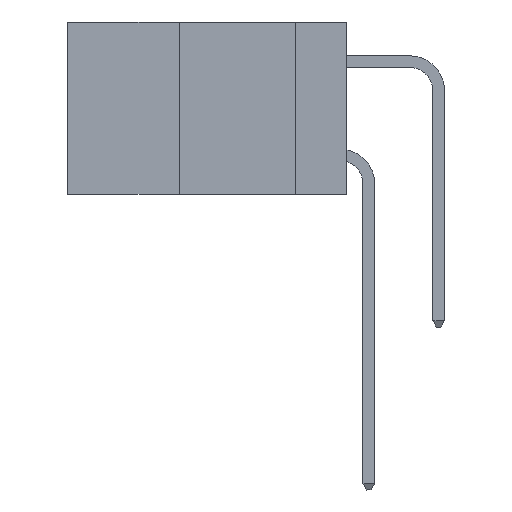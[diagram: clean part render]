
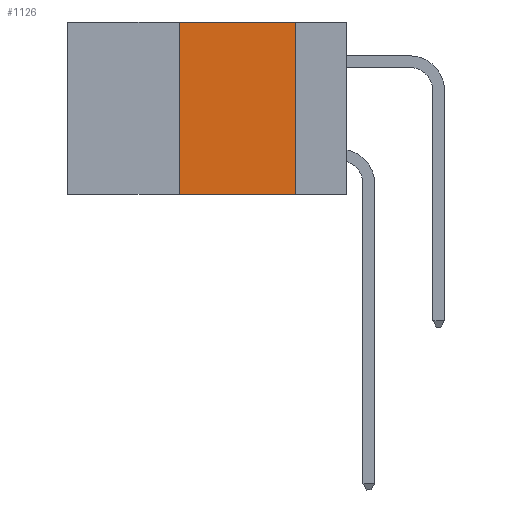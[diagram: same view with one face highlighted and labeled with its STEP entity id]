
A CAD part, left-side view. The second image highlights one B-rep face of the part: STEP entity #1126.
In plain terms, the highlighted planar face has unit normal (-1, 0, 0).
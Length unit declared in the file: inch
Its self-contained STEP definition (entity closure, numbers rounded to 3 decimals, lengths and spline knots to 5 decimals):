
#387 = CARTESIAN_POINT ( 'NONE',  ( 0., 0.6, 0. ) ) ;
#1126 = ADVANCED_FACE ( 'NONE', ( #11434 ), #13312, .F. ) ;
#2024 = VERTEX_POINT ( 'NONE', #13563 ) ;
#3400 = CARTESIAN_POINT ( 'NONE',  ( 0., 0.36, -0.37 ) ) ;
#3711 = DIRECTION ( 'NONE',  ( 0., 0., -1. ) ) ;
#4154 = EDGE_CURVE ( 'NONE', #9058, #19935, #14479, .T. ) ;
#4183 = VECTOR ( 'NONE', #19944, 39.37008 ) ;
#4853 = CARTESIAN_POINT ( 'NONE',  ( 0., 0.6, 0. ) ) ;
#5461 = DIRECTION ( 'NONE',  ( 1., 0., 0. ) ) ;
#5566 = EDGE_LOOP ( 'NONE', ( #8523, #20035, #20902, #6973 ) ) ;
#5877 = VECTOR ( 'NONE', #8380, 39.37008 ) ;
#6034 = VECTOR ( 'NONE', #18378, 39.37008 ) ;
#6973 = ORIENTED_EDGE ( 'NONE', *, *, #12761, .T. ) ;
#8380 = DIRECTION ( 'NONE',  ( 0., 0., 1. ) ) ;
#8500 = CARTESIAN_POINT ( 'NONE',  ( 0., 0.36, 0. ) ) ;
#8523 = ORIENTED_EDGE ( 'NONE', *, *, #13667, .F. ) ;
#8695 = LINE ( 'NONE', #387, #4183 ) ;
#9058 = VERTEX_POINT ( 'NONE', #3400 ) ;
#11434 = FACE_OUTER_BOUND ( 'NONE', #5566, .T. ) ;
#12340 = EDGE_CURVE ( 'NONE', #19935, #2024, #8695, .T. ) ;
#12685 = CARTESIAN_POINT ( 'NONE',  ( 0., 0.11, -0.37 ) ) ;
#12761 = EDGE_CURVE ( 'NONE', #9058, #17149, #17138, .T. ) ;
#13045 = DIRECTION ( 'NONE',  ( 0., -1., 0. ) ) ;
#13312 = PLANE ( 'NONE',  #15324 ) ;
#13563 = CARTESIAN_POINT ( 'NONE',  ( 0., 0.11, 0. ) ) ;
#13667 = EDGE_CURVE ( 'NONE', #2024, #17149, #18321, .T. ) ;
#14479 = LINE ( 'NONE', #8500, #5877 ) ;
#15232 = CARTESIAN_POINT ( 'NONE',  ( 0., 0.36, 0. ) ) ;
#15324 = AXIS2_PLACEMENT_3D ( 'NONE', #4853, #5461, #3711 ) ;
#16208 = CARTESIAN_POINT ( 'NONE',  ( 0., 0.6, -0.37 ) ) ;
#16637 = VECTOR ( 'NONE', #13045, 39.37008 ) ;
#16802 = CARTESIAN_POINT ( 'NONE',  ( 0., 0.11, 0. ) ) ;
#17138 = LINE ( 'NONE', #16208, #16637 ) ;
#17149 = VERTEX_POINT ( 'NONE', #12685 ) ;
#18321 = LINE ( 'NONE', #16802, #6034 ) ;
#18378 = DIRECTION ( 'NONE',  ( 0., 0., -1. ) ) ;
#19935 = VERTEX_POINT ( 'NONE', #15232 ) ;
#19944 = DIRECTION ( 'NONE',  ( 0., -1., 0. ) ) ;
#20035 = ORIENTED_EDGE ( 'NONE', *, *, #12340, .F. ) ;
#20902 = ORIENTED_EDGE ( 'NONE', *, *, #4154, .F. ) ;
